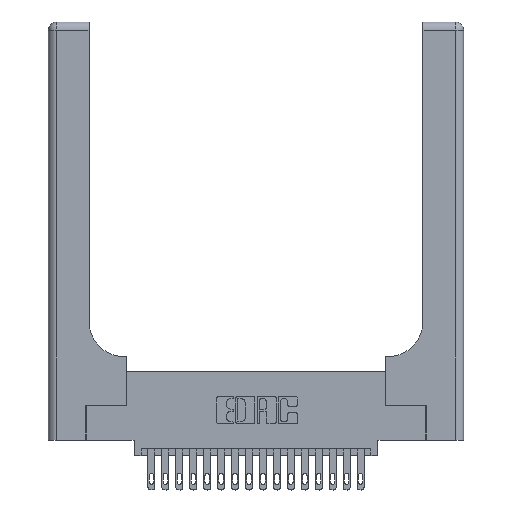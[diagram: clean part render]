
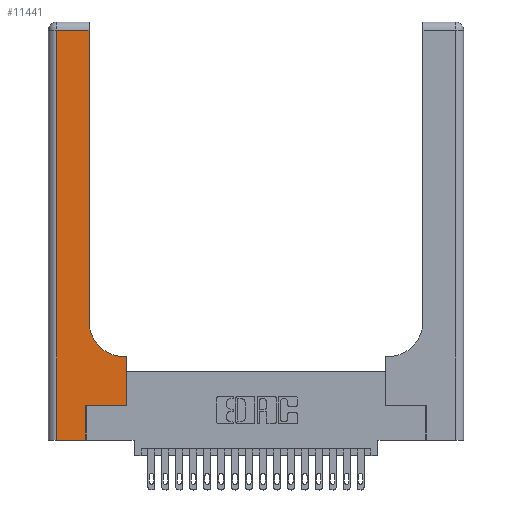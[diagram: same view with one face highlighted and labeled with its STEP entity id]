
A CAD part, top view. The second image highlights one B-rep face of the part: STEP entity #11441.
In plain terms, the highlighted planar face has unit normal (0, 0, 1).
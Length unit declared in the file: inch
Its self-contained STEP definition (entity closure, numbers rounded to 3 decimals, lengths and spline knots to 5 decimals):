
#1147 = CARTESIAN_POINT ( 'NONE',  ( 0.5585, 0.6, 0.37 ) ) ;
#1152 = VECTOR ( 'NONE', #12284, 39.37008 ) ;
#1201 = CARTESIAN_POINT ( 'NONE',  ( 0.06, 3., 0.37 ) ) ;
#1814 = CARTESIAN_POINT ( 'NONE',  ( 0.269, 0.25, 0.37 ) ) ;
#2603 = AXIS2_PLACEMENT_3D ( 'NONE', #20628, #14278, #7547 ) ;
#2782 = CARTESIAN_POINT ( 'NONE',  ( 0., 3., 0.37 ) ) ;
#3344 = VERTEX_POINT ( 'NONE', #20112 ) ;
#3537 = VECTOR ( 'NONE', #18090, 39.37008 ) ;
#3606 = EDGE_CURVE ( 'NONE', #17022, #3344, #3792, .T. ) ;
#3792 = LINE ( 'NONE', #18124, #20801 ) ;
#4397 = LINE ( 'NONE', #18539, #10312 ) ;
#4410 = FACE_OUTER_BOUND ( 'NONE', #7179, .T. ) ;
#4420 = DIRECTION ( 'NONE',  ( -1., 0., 0. ) ) ;
#4421 = VECTOR ( 'NONE', #14541, 39.37008 ) ;
#4513 = LINE ( 'NONE', #5880, #1152 ) ;
#4869 = EDGE_CURVE ( 'NONE', #3344, #10398, #9422, .T. ) ;
#4966 = EDGE_CURVE ( 'NONE', #13154, #14519, #4513, .T. ) ;
#5176 = ORIENTED_EDGE ( 'NONE', *, *, #4869, .T. ) ;
#5191 = EDGE_CURVE ( 'NONE', #10199, #20697, #6579, .T. ) ;
#5803 = PLANE ( 'NONE',  #11838 ) ;
#5818 = VECTOR ( 'NONE', #19187, 39.37008 ) ;
#5880 = CARTESIAN_POINT ( 'NONE',  ( 0.269, 0., 0.37 ) ) ;
#6579 = LINE ( 'NONE', #15040, #20979 ) ;
#7179 = EDGE_LOOP ( 'NONE', ( #20786, #8590, #5176, #19627, #14034, #19345, #10334, #9024, #14138 ) ) ;
#7439 = DIRECTION ( 'NONE',  ( 1., 0., 0. ) ) ;
#7547 = DIRECTION ( 'NONE',  ( 1., 0., 0. ) ) ;
#7861 = CIRCLE ( 'NONE', #2603, 0.25 ) ;
#8208 = CARTESIAN_POINT ( 'NONE',  ( 0.06, 0., 0.37 ) ) ;
#8270 = EDGE_CURVE ( 'NONE', #10398, #13154, #8795, .T. ) ;
#8590 = ORIENTED_EDGE ( 'NONE', *, *, #3606, .T. ) ;
#8795 = LINE ( 'NONE', #9013, #18044 ) ;
#9013 = CARTESIAN_POINT ( 'NONE',  ( 0., 0., 0.37 ) ) ;
#9024 = ORIENTED_EDGE ( 'NONE', *, *, #5191, .T. ) ;
#9293 = DIRECTION ( 'NONE',  ( -1., 0., 0. ) ) ;
#9422 = LINE ( 'NONE', #1201, #5818 ) ;
#9457 = EDGE_CURVE ( 'NONE', #20697, #20701, #7861, .T. ) ;
#10199 = VERTEX_POINT ( 'NONE', #1147 ) ;
#10312 = VECTOR ( 'NONE', #15086, 39.37008 ) ;
#10334 = ORIENTED_EDGE ( 'NONE', *, *, #20053, .T. ) ;
#10398 = VERTEX_POINT ( 'NONE', #8208 ) ;
#10973 = CARTESIAN_POINT ( 'NONE',  ( 0.5415, 0.6, 0.37 ) ) ;
#11020 = DIRECTION ( 'NONE',  ( 0., 0., -1. ) ) ;
#11441 = ADVANCED_FACE ( 'NONE', ( #4410 ), #5803, .F. ) ;
#11838 = AXIS2_PLACEMENT_3D ( 'NONE', #2782, #11020, #4420 ) ;
#12284 = DIRECTION ( 'NONE',  ( 0., 1., 0. ) ) ;
#13154 = VERTEX_POINT ( 'NONE', #19395 ) ;
#13290 = EDGE_CURVE ( 'NONE', #14519, #20456, #16399, .T. ) ;
#14034 = ORIENTED_EDGE ( 'NONE', *, *, #4966, .T. ) ;
#14138 = ORIENTED_EDGE ( 'NONE', *, *, #9457, .T. ) ;
#14278 = DIRECTION ( 'NONE',  ( 0., 0., -1. ) ) ;
#14519 = VERTEX_POINT ( 'NONE', #20800 ) ;
#14541 = DIRECTION ( 'NONE',  ( 0., 1., 0. ) ) ;
#14947 = LINE ( 'NONE', #17586, #4421 ) ;
#15040 = CARTESIAN_POINT ( 'NONE',  ( 0.2915, 0.6, 0.37 ) ) ;
#15086 = DIRECTION ( 'NONE',  ( 0., 1., 0. ) ) ;
#16399 = LINE ( 'NONE', #1814, #3537 ) ;
#17022 = VERTEX_POINT ( 'NONE', #20525 ) ;
#17551 = CARTESIAN_POINT ( 'NONE',  ( 0.2915, 0.85, 0.37 ) ) ;
#17586 = CARTESIAN_POINT ( 'NONE',  ( 0.5585, 0.25, 0.37 ) ) ;
#17993 = DIRECTION ( 'NONE',  ( -1., 0., 0. ) ) ;
#18044 = VECTOR ( 'NONE', #7439, 39.37008 ) ;
#18090 = DIRECTION ( 'NONE',  ( 1., 0., 0. ) ) ;
#18124 = CARTESIAN_POINT ( 'NONE',  ( 0., 2.94, 0.37 ) ) ;
#18539 = CARTESIAN_POINT ( 'NONE',  ( 0.2915, 3., 0.37 ) ) ;
#19187 = DIRECTION ( 'NONE',  ( 0., -1., 0. ) ) ;
#19345 = ORIENTED_EDGE ( 'NONE', *, *, #13290, .T. ) ;
#19395 = CARTESIAN_POINT ( 'NONE',  ( 0.269, 0., 0.37 ) ) ;
#19627 = ORIENTED_EDGE ( 'NONE', *, *, #8270, .T. ) ;
#20053 = EDGE_CURVE ( 'NONE', #20456, #10199, #14947, .T. ) ;
#20112 = CARTESIAN_POINT ( 'NONE',  ( 0.06, 2.94, 0.37 ) ) ;
#20271 = CARTESIAN_POINT ( 'NONE',  ( 0.5585, 0.25, 0.37 ) ) ;
#20335 = EDGE_CURVE ( 'NONE', #20701, #17022, #4397, .T. ) ;
#20456 = VERTEX_POINT ( 'NONE', #20271 ) ;
#20525 = CARTESIAN_POINT ( 'NONE',  ( 0.2915, 2.94, 0.37 ) ) ;
#20628 = CARTESIAN_POINT ( 'NONE',  ( 0.5415, 0.85, 0.37 ) ) ;
#20697 = VERTEX_POINT ( 'NONE', #10973 ) ;
#20701 = VERTEX_POINT ( 'NONE', #17551 ) ;
#20786 = ORIENTED_EDGE ( 'NONE', *, *, #20335, .T. ) ;
#20800 = CARTESIAN_POINT ( 'NONE',  ( 0.269, 0.25, 0.37 ) ) ;
#20801 = VECTOR ( 'NONE', #17993, 39.37008 ) ;
#20979 = VECTOR ( 'NONE', #9293, 39.37008 ) ;
